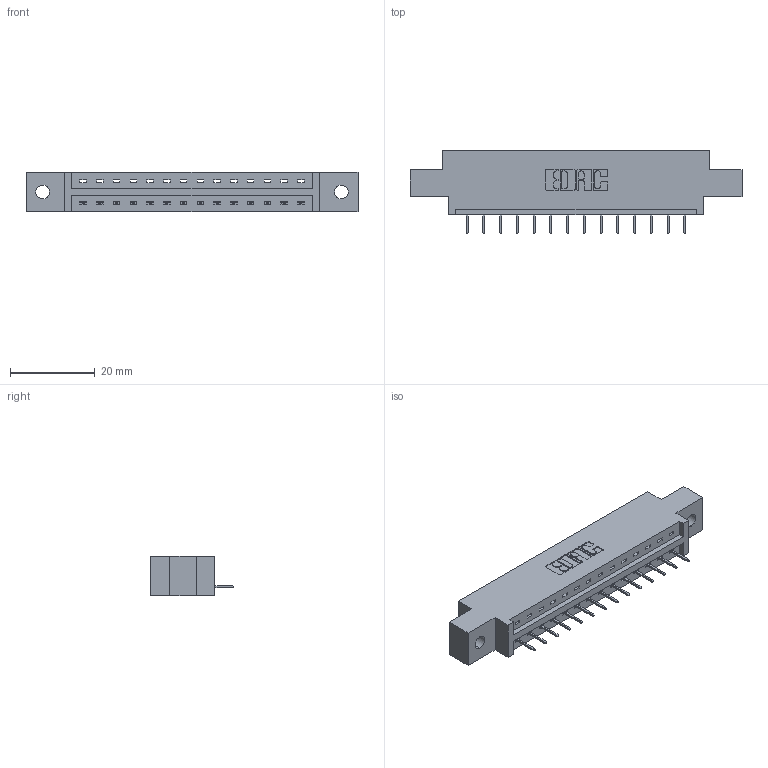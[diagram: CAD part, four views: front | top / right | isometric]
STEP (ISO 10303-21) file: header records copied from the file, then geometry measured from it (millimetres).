
FILE_DESCRIPTION (( 'STEP AP203' ), '1' );
FILE_NAME ('337-014-524-602.STEP', '2019-09-28T15:40:15', ( '' ), ( '' ), 'SwSTEP 2.0', 'SolidWorks 2016', '' );
FILE_SCHEMA (( 'CONFIG_CONTROL_DESIGN' ));
Length unit declared in the file: inch
Products named in the file (3): 337-014-524-602; 345-292-001_345-293-124; 337 Part_0.170 Offset - 0.128 Dia
Assembly tree (15 placements, depth 2):
  337-014-524-602
    337 Part_0.170 Offset - 0.128 Dia
    345-292-001_345-293-124  x14
Bounding box: 78.49 x 19.69 x 9.4 mm (x, y, z)
Volume: 7597.4 mm3; surface area: 7327.5 mm2
Topology: 15 solids, 15 shells, 1042 faces, 3011 edges, 1950 vertices
Faces by surface type: plane 802, cylinder 240
Entity records: 14237 total; most frequent: CARTESIAN_POINT 2484, ORIENTED_EDGE 2434, DIRECTION 2149, EDGE_CURVE 1217, LINE 1093, VECTOR 1093, VERTEX_POINT 806, AXIS2_PLACEMENT_3D 528
